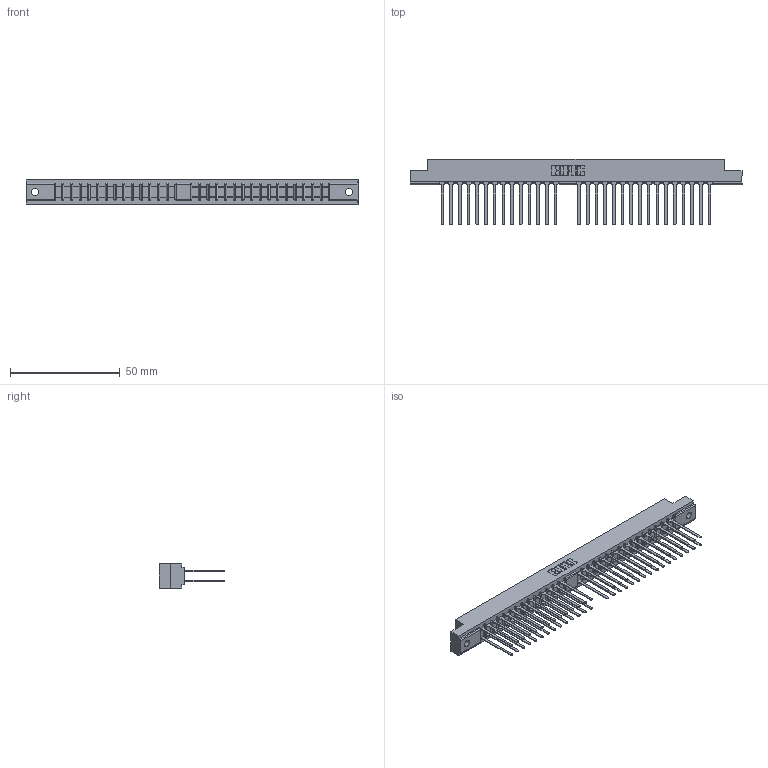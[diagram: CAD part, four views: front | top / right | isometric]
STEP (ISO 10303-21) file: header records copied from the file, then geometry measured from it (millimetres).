
FILE_DESCRIPTION (( 'STEP AP203' ), '1' );
FILE_NAME ('310-060-540-202.STEP', '2020-03-25T13:59:15', ( '' ), ( '' ), 'SwSTEP 2.0', 'SolidWorks 2016', '' );
FILE_SCHEMA (( 'CONFIG_CONTROL_DESIGN' ));
Length unit declared in the file: millimetre
Products named in the file (3): 307-290-001_540; 310 Part_.128 Dia. Hole; 310-060-540-202
Assembly tree (61 placements, depth 2):
  310-060-540-202
    310 Part_.128 Dia. Hole
    307-290-001_540  x60
Bounding box: 151.21 x 29.95 x 10.97 mm (x, y, z)
Volume: 13308.8 mm3; surface area: 19872.2 mm2
Topology: 61 solids, 61 shells, 2926 faces, 8161 edges, 5270 vertices
Faces by surface type: plane 1944, cylinder 918, sphere 64
Entity records: 28554 total; most frequent: CARTESIAN_POINT 4675, ORIENTED_EDGE 4630, DIRECTION 4585, EDGE_CURVE 2315, VECTOR 1777, LINE 1777, VERTEX_POINT 1494, AXIS2_PLACEMENT_3D 1404
